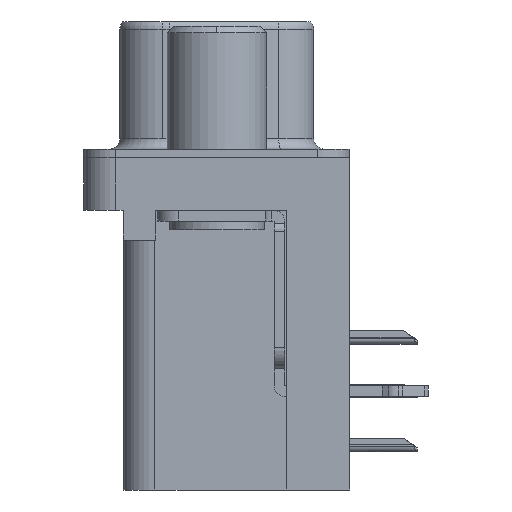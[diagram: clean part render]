
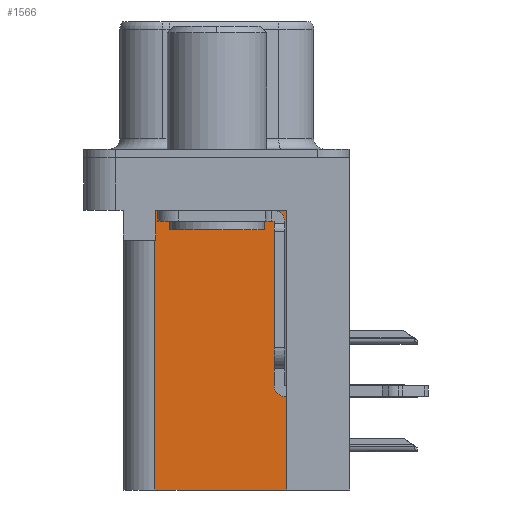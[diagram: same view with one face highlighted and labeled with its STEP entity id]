
A CAD part, left-side view. The second image highlights one B-rep face of the part: STEP entity #1566.
In plain terms, the highlighted planar face has unit normal (-1, 0, 0).
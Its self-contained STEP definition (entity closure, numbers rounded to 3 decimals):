
#1566 = ADVANCED_FACE ( 'NONE', ( #10558 ), #1627, .F. ) ;
#1627 = PLANE ( 'NONE',  #22739 ) ;
#1935 = EDGE_CURVE ( 'NONE', #29964, #7673, #20440, .T. ) ;
#2634 = DIRECTION ( 'NONE',  ( 0., 0., 1. ) ) ;
#3128 = CARTESIAN_POINT ( 'NONE',  ( 3.7, -3.295, -15.7 ) ) ;
#3824 = DIRECTION ( 'NONE',  ( 1., 0., 0. ) ) ;
#3904 = VERTEX_POINT ( 'NONE', #10521 ) ;
#3929 = DIRECTION ( 'NONE',  ( 0., 0., -1. ) ) ;
#4141 = CARTESIAN_POINT ( 'NONE',  ( 3.7, 2.895, -3.9 ) ) ;
#4330 = VECTOR ( 'NONE', #2634, 1000. ) ;
#6066 = CARTESIAN_POINT ( 'NONE',  ( 3.7, 0., -3.9 ) ) ;
#6306 = ORIENTED_EDGE ( 'NONE', *, *, #26584, .T. ) ;
#6679 = VECTOR ( 'NONE', #7655, 1000. ) ;
#6851 = CARTESIAN_POINT ( 'NONE',  ( 3.7, 2.925, -15.7 ) ) ;
#7655 = DIRECTION ( 'NONE',  ( 0., 1., 0. ) ) ;
#7673 = VERTEX_POINT ( 'NONE', #8890 ) ;
#7724 = VERTEX_POINT ( 'NONE', #6851 ) ;
#8221 = CARTESIAN_POINT ( 'NONE',  ( 3.7, 2.895, -3.9 ) ) ;
#8837 = EDGE_CURVE ( 'NONE', #7673, #13508, #16078, .T. ) ;
#8890 = CARTESIAN_POINT ( 'NONE',  ( 3.7, 2.895, -2.5 ) ) ;
#9761 = EDGE_CURVE ( 'NONE', #7724, #22308, #16759, .T. ) ;
#9969 = CARTESIAN_POINT ( 'NONE',  ( 3.7, -3.295, -15.7 ) ) ;
#10521 = CARTESIAN_POINT ( 'NONE',  ( 3.7, -3.295, -15.7 ) ) ;
#10558 = FACE_OUTER_BOUND ( 'NONE', #13201, .T. ) ;
#11782 = VECTOR ( 'NONE', #16171, 1000. ) ;
#13201 = EDGE_LOOP ( 'NONE', ( #24693, #29305, #24016, #28594, #16211, #6306 ) ) ;
#13503 = CARTESIAN_POINT ( 'NONE',  ( 3.7, -3.295, -2.5 ) ) ;
#13508 = VERTEX_POINT ( 'NONE', #4141 ) ;
#13647 = LINE ( 'NONE', #6066, #14382 ) ;
#14204 = VECTOR ( 'NONE', #30352, 1000. ) ;
#14382 = VECTOR ( 'NONE', #24747, 1000. ) ;
#15365 = DIRECTION ( 'NONE',  ( 0., 0., -1. ) ) ;
#16078 = LINE ( 'NONE', #8221, #29322 ) ;
#16171 = DIRECTION ( 'NONE',  ( 0., 0., 1. ) ) ;
#16211 = ORIENTED_EDGE ( 'NONE', *, *, #16977, .F. ) ;
#16759 = LINE ( 'NONE', #23579, #4330 ) ;
#16977 = EDGE_CURVE ( 'NONE', #3904, #7724, #25290, .T. ) ;
#18047 = LINE ( 'NONE', #25442, #11782 ) ;
#20260 = EDGE_CURVE ( 'NONE', #13508, #22308, #13647, .T. ) ;
#20440 = LINE ( 'NONE', #25522, #14204 ) ;
#22308 = VERTEX_POINT ( 'NONE', #23110 ) ;
#22739 = AXIS2_PLACEMENT_3D ( 'NONE', #3128, #3824, #3929 ) ;
#23110 = CARTESIAN_POINT ( 'NONE',  ( 3.7, 2.925, -3.9 ) ) ;
#23579 = CARTESIAN_POINT ( 'NONE',  ( 3.7, 2.925, -15.7 ) ) ;
#24016 = ORIENTED_EDGE ( 'NONE', *, *, #20260, .T. ) ;
#24693 = ORIENTED_EDGE ( 'NONE', *, *, #1935, .T. ) ;
#24747 = DIRECTION ( 'NONE',  ( 0., 1., 0. ) ) ;
#25290 = LINE ( 'NONE', #9969, #6679 ) ;
#25442 = CARTESIAN_POINT ( 'NONE',  ( 3.7, -3.295, -15.7 ) ) ;
#25522 = CARTESIAN_POINT ( 'NONE',  ( 3.7, -3.295, -2.5 ) ) ;
#26584 = EDGE_CURVE ( 'NONE', #3904, #29964, #18047, .T. ) ;
#28594 = ORIENTED_EDGE ( 'NONE', *, *, #9761, .F. ) ;
#29305 = ORIENTED_EDGE ( 'NONE', *, *, #8837, .T. ) ;
#29322 = VECTOR ( 'NONE', #15365, 1000. ) ;
#29964 = VERTEX_POINT ( 'NONE', #13503 ) ;
#30352 = DIRECTION ( 'NONE',  ( 0., 1., 0. ) ) ;
